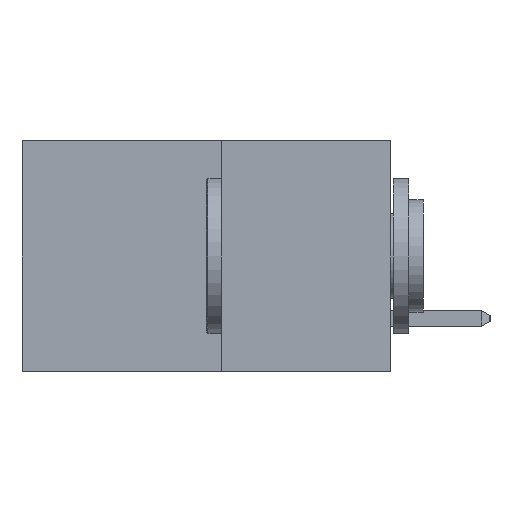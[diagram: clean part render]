
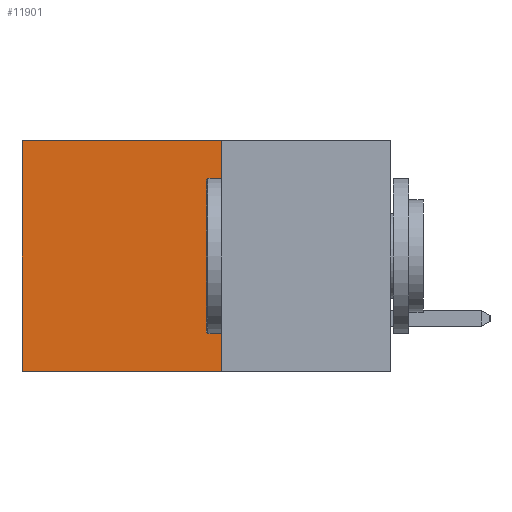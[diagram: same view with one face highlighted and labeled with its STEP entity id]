
A CAD part, left-side view. The second image highlights one B-rep face of the part: STEP entity #11901.
In plain terms, the highlighted planar face has unit normal (-1, 0, 0).
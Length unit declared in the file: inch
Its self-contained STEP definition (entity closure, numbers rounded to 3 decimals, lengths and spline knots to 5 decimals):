
#220 = DIRECTION ( 'NONE',  ( 0., 0., -1. ) ) ;
#644 = VECTOR ( 'NONE', #2331, 39.37008 ) ;
#712 = DIRECTION ( 'NONE',  ( 0., 1., 0. ) ) ;
#2331 = DIRECTION ( 'NONE',  ( 0., 0., -1. ) ) ;
#2547 = DIRECTION ( 'NONE',  ( 0., 0., -1. ) ) ;
#3541 = VERTEX_POINT ( 'NONE', #12937 ) ;
#3572 = FACE_OUTER_BOUND ( 'NONE', #18922, .T. ) ;
#4058 = CARTESIAN_POINT ( 'NONE',  ( 0.277, 0.59, 0. ) ) ;
#4078 = VECTOR ( 'NONE', #712, 39.37008 ) ;
#4532 = VECTOR ( 'NONE', #21097, 39.37008 ) ;
#4651 = LINE ( 'NONE', #16730, #4078 ) ;
#5657 = VERTEX_POINT ( 'NONE', #11696 ) ;
#5832 = VERTEX_POINT ( 'NONE', #8956 ) ;
#7254 = EDGE_CURVE ( 'NONE', #3541, #17456, #4651, .T. ) ;
#7329 = CARTESIAN_POINT ( 'NONE',  ( 0.277, 0.27, -0.37 ) ) ;
#8794 = CARTESIAN_POINT ( 'NONE',  ( 0.277, 0.27, -0.37 ) ) ;
#8956 = CARTESIAN_POINT ( 'NONE',  ( 0.277, 0.59, -0.37 ) ) ;
#9090 = PLANE ( 'NONE',  #9285 ) ;
#9285 = AXIS2_PLACEMENT_3D ( 'NONE', #7329, #10940, #220 ) ;
#9391 = ORIENTED_EDGE ( 'NONE', *, *, #7254, .T. ) ;
#10940 = DIRECTION ( 'NONE',  ( 1., 0., 0. ) ) ;
#11030 = VECTOR ( 'NONE', #2547, 39.37008 ) ;
#11357 = ORIENTED_EDGE ( 'NONE', *, *, #22834, .T. ) ;
#11696 = CARTESIAN_POINT ( 'NONE',  ( 0.277, 0.27, -0.37 ) ) ;
#11901 = ADVANCED_FACE ( 'NONE', ( #3572 ), #9090, .F. ) ;
#12937 = CARTESIAN_POINT ( 'NONE',  ( 0.277, 0.27, 0. ) ) ;
#13090 = EDGE_CURVE ( 'NONE', #3541, #5657, #16297, .T. ) ;
#13469 = LINE ( 'NONE', #8794, #4532 ) ;
#15024 = CARTESIAN_POINT ( 'NONE',  ( 0.277, 0.27, -0.37 ) ) ;
#16297 = LINE ( 'NONE', #15024, #11030 ) ;
#16569 = CARTESIAN_POINT ( 'NONE',  ( 0.277, 0.59, -0.37 ) ) ;
#16730 = CARTESIAN_POINT ( 'NONE',  ( 0.277, 0.27, 0. ) ) ;
#17456 = VERTEX_POINT ( 'NONE', #4058 ) ;
#18922 = EDGE_LOOP ( 'NONE', ( #11357, #20903, #20377, #9391 ) ) ;
#19104 = EDGE_CURVE ( 'NONE', #5657, #5832, #13469, .T. ) ;
#19460 = LINE ( 'NONE', #16569, #644 ) ;
#20377 = ORIENTED_EDGE ( 'NONE', *, *, #13090, .F. ) ;
#20903 = ORIENTED_EDGE ( 'NONE', *, *, #19104, .F. ) ;
#21097 = DIRECTION ( 'NONE',  ( 0., 1., 0. ) ) ;
#22834 = EDGE_CURVE ( 'NONE', #17456, #5832, #19460, .T. ) ;
